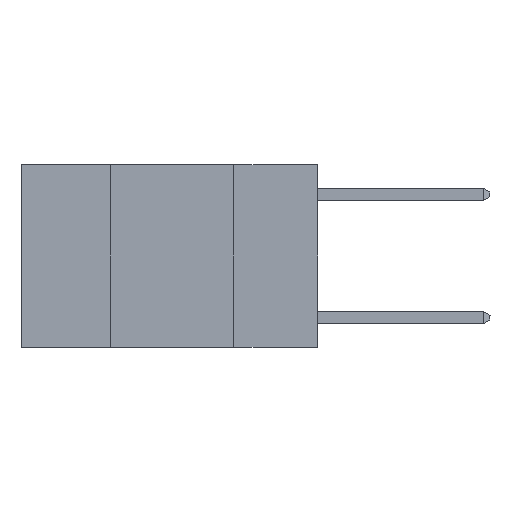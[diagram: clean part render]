
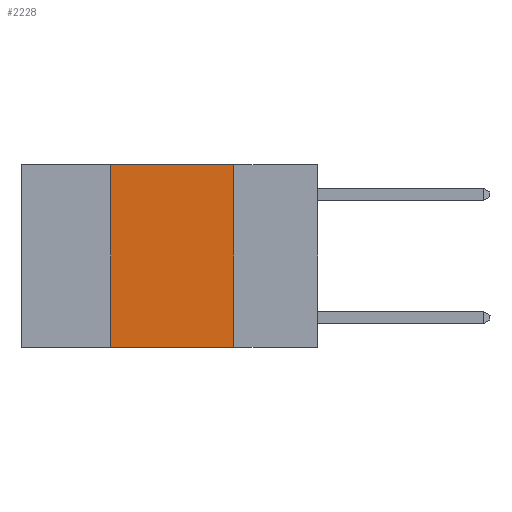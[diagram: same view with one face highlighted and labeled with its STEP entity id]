
A CAD part, left-side view. The second image highlights one B-rep face of the part: STEP entity #2228.
In plain terms, the highlighted planar face has unit normal (-1, 0, 0).
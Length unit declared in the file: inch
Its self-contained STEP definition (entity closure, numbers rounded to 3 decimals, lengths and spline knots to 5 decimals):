
#511 = DIRECTION ( 'NONE',  ( 0., 0., 1. ) ) ;
#1675 = ORIENTED_EDGE ( 'NONE', *, *, #14901, .F. ) ;
#2228 = ADVANCED_FACE ( 'NONE', ( #6807 ), #4108, .F. ) ;
#2242 = ORIENTED_EDGE ( 'NONE', *, *, #18746, .F. ) ;
#2802 = ORIENTED_EDGE ( 'NONE', *, *, #13498, .F. ) ;
#3644 = ORIENTED_EDGE ( 'NONE', *, *, #14998, .T. ) ;
#4108 = PLANE ( 'NONE',  #18989 ) ;
#4420 = DIRECTION ( 'NONE',  ( 0., -1., 0. ) ) ;
#6644 = CARTESIAN_POINT ( 'NONE',  ( 0., 0.17, 0. ) ) ;
#6807 = FACE_OUTER_BOUND ( 'NONE', #20706, .T. ) ;
#7342 = CARTESIAN_POINT ( 'NONE',  ( 0., 0.17, -0.37 ) ) ;
#7685 = VECTOR ( 'NONE', #511, 39.37008 ) ;
#8068 = VERTEX_POINT ( 'NONE', #23220 ) ;
#10409 = VERTEX_POINT ( 'NONE', #21042 ) ;
#10597 = VECTOR ( 'NONE', #4420, 39.37008 ) ;
#10717 = VECTOR ( 'NONE', #29049, 39.37008 ) ;
#11311 = LINE ( 'NONE', #29542, #10597 ) ;
#13498 = EDGE_CURVE ( 'NONE', #8068, #10409, #13946, .T. ) ;
#13946 = LINE ( 'NONE', #25955, #7685 ) ;
#14901 = EDGE_CURVE ( 'NONE', #22079, #27453, #19515, .T. ) ;
#14998 = EDGE_CURVE ( 'NONE', #8068, #27453, #11311, .T. ) ;
#15916 = DIRECTION ( 'NONE',  ( 0., 0., -1. ) ) ;
#18746 = EDGE_CURVE ( 'NONE', #10409, #22079, #22081, .T. ) ;
#18809 = VECTOR ( 'NONE', #20456, 39.37008 ) ;
#18989 = AXIS2_PLACEMENT_3D ( 'NONE', #22583, #29350, #15916 ) ;
#19515 = LINE ( 'NONE', #6644, #18809 ) ;
#20049 = CARTESIAN_POINT ( 'NONE',  ( 0., 0.6, 0. ) ) ;
#20456 = DIRECTION ( 'NONE',  ( 0., 0., -1. ) ) ;
#20706 = EDGE_LOOP ( 'NONE', ( #1675, #2242, #2802, #3644 ) ) ;
#21042 = CARTESIAN_POINT ( 'NONE',  ( 0., 0.42, 0. ) ) ;
#22079 = VERTEX_POINT ( 'NONE', #22184 ) ;
#22081 = LINE ( 'NONE', #20049, #10717 ) ;
#22184 = CARTESIAN_POINT ( 'NONE',  ( 0., 0.17, 0. ) ) ;
#22583 = CARTESIAN_POINT ( 'NONE',  ( 0., 0.6, 0. ) ) ;
#23220 = CARTESIAN_POINT ( 'NONE',  ( 0., 0.42, -0.37 ) ) ;
#25955 = CARTESIAN_POINT ( 'NONE',  ( 0., 0.42, 0. ) ) ;
#27453 = VERTEX_POINT ( 'NONE', #7342 ) ;
#29049 = DIRECTION ( 'NONE',  ( 0., -1., 0. ) ) ;
#29350 = DIRECTION ( 'NONE',  ( 1., 0., 0. ) ) ;
#29542 = CARTESIAN_POINT ( 'NONE',  ( 0., 0.6, -0.37 ) ) ;
